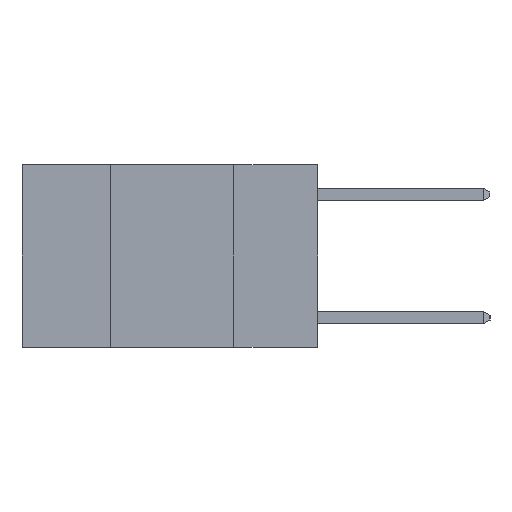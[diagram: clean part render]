
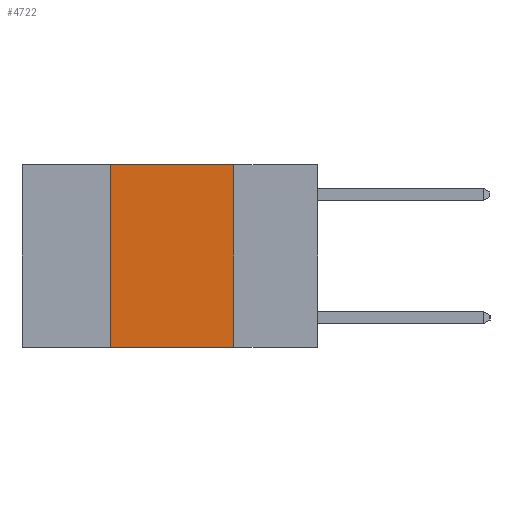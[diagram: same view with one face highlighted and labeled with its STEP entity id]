
A CAD part, left-side view. The second image highlights one B-rep face of the part: STEP entity #4722.
In plain terms, the highlighted planar face has unit normal (-1, 0, 0).
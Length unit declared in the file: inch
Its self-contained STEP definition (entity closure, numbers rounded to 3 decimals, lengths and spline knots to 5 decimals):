
#587 = ORIENTED_EDGE ( 'NONE', *, *, #3204, .F. ) ;
#1087 = DIRECTION ( 'NONE',  ( 0., 0., -1. ) ) ;
#1506 = PLANE ( 'NONE',  #3538 ) ;
#1524 = VERTEX_POINT ( 'NONE', #5693 ) ;
#1577 = DIRECTION ( 'NONE',  ( 0., -1., 0. ) ) ;
#1933 = CARTESIAN_POINT ( 'NONE',  ( 0., 0.6, -0.37 ) ) ;
#1988 = VECTOR ( 'NONE', #1087, 39.37008 ) ;
#2330 = CARTESIAN_POINT ( 'NONE',  ( 0., 0.17, 0. ) ) ;
#2356 = DIRECTION ( 'NONE',  ( 1., 0., 0. ) ) ;
#3031 = CARTESIAN_POINT ( 'NONE',  ( 0., 0.42, 0. ) ) ;
#3204 = EDGE_CURVE ( 'NONE', #10576, #3802, #6080, .T. ) ;
#3282 = CARTESIAN_POINT ( 'NONE',  ( 0., 0.6, 0. ) ) ;
#3538 = AXIS2_PLACEMENT_3D ( 'NONE', #6418, #2356, #8043 ) ;
#3802 = VERTEX_POINT ( 'NONE', #4334 ) ;
#4334 = CARTESIAN_POINT ( 'NONE',  ( 0., 0.17, -0.37 ) ) ;
#4571 = VERTEX_POINT ( 'NONE', #9342 ) ;
#4722 = ADVANCED_FACE ( 'NONE', ( #10107 ), #1506, .F. ) ;
#4908 = VECTOR ( 'NONE', #5239, 39.37008 ) ;
#5014 = EDGE_CURVE ( 'NONE', #1524, #3802, #7041, .T. ) ;
#5239 = DIRECTION ( 'NONE',  ( 0., -1., 0. ) ) ;
#5374 = LINE ( 'NONE', #3031, #9423 ) ;
#5693 = CARTESIAN_POINT ( 'NONE',  ( 0., 0.42, -0.37 ) ) ;
#5865 = ORIENTED_EDGE ( 'NONE', *, *, #5014, .T. ) ;
#6080 = LINE ( 'NONE', #10077, #1988 ) ;
#6418 = CARTESIAN_POINT ( 'NONE',  ( 0., 0.6, 0. ) ) ;
#7041 = LINE ( 'NONE', #1933, #4908 ) ;
#7046 = DIRECTION ( 'NONE',  ( 0., 0., 1. ) ) ;
#7417 = EDGE_CURVE ( 'NONE', #1524, #4571, #5374, .T. ) ;
#7959 = LINE ( 'NONE', #3282, #9602 ) ;
#8043 = DIRECTION ( 'NONE',  ( 0., 0., -1. ) ) ;
#8336 = EDGE_LOOP ( 'NONE', ( #587, #10594, #9271, #5865 ) ) ;
#9271 = ORIENTED_EDGE ( 'NONE', *, *, #7417, .F. ) ;
#9342 = CARTESIAN_POINT ( 'NONE',  ( 0., 0.42, 0. ) ) ;
#9423 = VECTOR ( 'NONE', #7046, 39.37008 ) ;
#9602 = VECTOR ( 'NONE', #1577, 39.37008 ) ;
#10008 = EDGE_CURVE ( 'NONE', #4571, #10576, #7959, .T. ) ;
#10077 = CARTESIAN_POINT ( 'NONE',  ( 0., 0.17, 0. ) ) ;
#10107 = FACE_OUTER_BOUND ( 'NONE', #8336, .T. ) ;
#10576 = VERTEX_POINT ( 'NONE', #2330 ) ;
#10594 = ORIENTED_EDGE ( 'NONE', *, *, #10008, .F. ) ;
